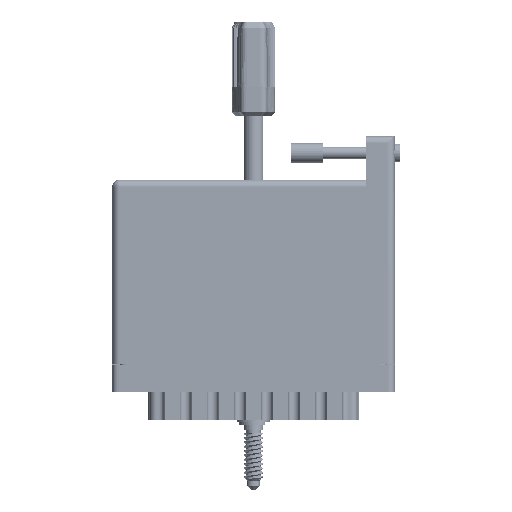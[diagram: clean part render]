
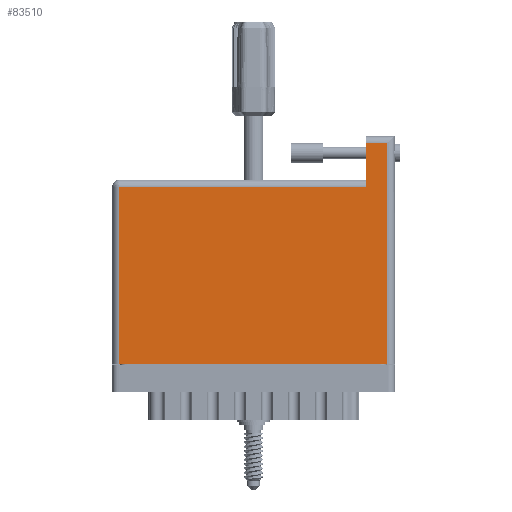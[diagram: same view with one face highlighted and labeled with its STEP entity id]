
A CAD part, front view. The second image highlights one B-rep face of the part: STEP entity #83510.
In plain terms, the highlighted face is planar.
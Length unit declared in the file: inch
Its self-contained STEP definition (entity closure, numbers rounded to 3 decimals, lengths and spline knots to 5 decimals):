
#1133 = VECTOR ( 'NONE', #14040, 39.37008 ) ;
#1445 = CARTESIAN_POINT ( 'NONE',  ( 0.07, 1.705, 0. ) ) ;
#1449 = CARTESIAN_POINT ( 'NONE',  ( 0., 1.775, 0. ) ) ;
#6868 = EDGE_CURVE ( 'NONE', #33301, #13850, #14302, .T. ) ;
#8871 = AXIS2_PLACEMENT_3D ( 'NONE', #1449, #35741, #36329 ) ;
#9872 = LINE ( 'NONE', #56781, #33595 ) ;
#11397 = VECTOR ( 'NONE', #49654, 39.37008 ) ;
#13599 = CARTESIAN_POINT ( 'NONE',  ( 2.438, 2.195, 0. ) ) ;
#13850 = VERTEX_POINT ( 'NONE', #48962 ) ;
#14040 = DIRECTION ( 'NONE',  ( -1., 0., 0. ) ) ;
#14302 = LINE ( 'NONE', #68825, #68151 ) ;
#14479 = EDGE_CURVE ( 'NONE', #65172, #54141, #22150, .T. ) ;
#15605 = ORIENTED_EDGE ( 'NONE', *, *, #6868, .T. ) ;
#17155 = EDGE_CURVE ( 'NONE', #54141, #33301, #9872, .T. ) ;
#19374 = DIRECTION ( 'NONE',  ( 0., 1., 0. ) ) ;
#20775 = ORIENTED_EDGE ( 'NONE', *, *, #49079, .T. ) ;
#22150 = LINE ( 'NONE', #13599, #11397 ) ;
#22291 = ORIENTED_EDGE ( 'NONE', *, *, #17155, .T. ) ;
#32911 = CARTESIAN_POINT ( 'NONE',  ( 2.438, 1.705, 0. ) ) ;
#33004 = ORIENTED_EDGE ( 'NONE', *, *, #87401, .T. ) ;
#33038 = CARTESIAN_POINT ( 'NONE',  ( 2.648, 0., 0. ) ) ;
#33301 = VERTEX_POINT ( 'NONE', #1445 ) ;
#33422 = LINE ( 'NONE', #89007, #1133 ) ;
#33595 = VECTOR ( 'NONE', #64015, 39.37008 ) ;
#35741 = DIRECTION ( 'NONE',  ( 0., 0., -1. ) ) ;
#36329 = DIRECTION ( 'NONE',  ( -1., 0., 0. ) ) ;
#37536 = ORIENTED_EDGE ( 'NONE', *, *, #14479, .T. ) ;
#39173 = CARTESIAN_POINT ( 'NONE',  ( 2.438, 2.125, 0. ) ) ;
#39257 = DIRECTION ( 'NONE',  ( 1., 0., 0. ) ) ;
#43702 = EDGE_CURVE ( 'NONE', #71905, #65172, #33422, .T. ) ;
#46460 = FACE_OUTER_BOUND ( 'NONE', #63848, .T. ) ;
#47483 = LINE ( 'NONE', #61271, #85107 ) ;
#48962 = CARTESIAN_POINT ( 'NONE',  ( 0.07, 0., 0. ) ) ;
#49079 = EDGE_CURVE ( 'NONE', #64079, #71905, #47483, .T. ) ;
#49654 = DIRECTION ( 'NONE',  ( 0., -1., 0. ) ) ;
#53445 = CARTESIAN_POINT ( 'NONE',  ( 0., 0., 0. ) ) ;
#54141 = VERTEX_POINT ( 'NONE', #32911 ) ;
#55409 = CARTESIAN_POINT ( 'NONE',  ( 2.648, 2.125, 0. ) ) ;
#56781 = CARTESIAN_POINT ( 'NONE',  ( 0., 1.705, 0. ) ) ;
#61271 = CARTESIAN_POINT ( 'NONE',  ( 2.648, 2.195, 0. ) ) ;
#61623 = DIRECTION ( 'NONE',  ( 0., -1., 0. ) ) ;
#63848 = EDGE_LOOP ( 'NONE', ( #22291, #15605, #33004, #20775, #87727, #37536 ) ) ;
#64015 = DIRECTION ( 'NONE',  ( -1., 0., 0. ) ) ;
#64079 = VERTEX_POINT ( 'NONE', #33038 ) ;
#65172 = VERTEX_POINT ( 'NONE', #39173 ) ;
#66439 = VECTOR ( 'NONE', #39257, 39.37008 ) ;
#68151 = VECTOR ( 'NONE', #61623, 39.37008 ) ;
#68825 = CARTESIAN_POINT ( 'NONE',  ( 0.07, 0., 0. ) ) ;
#70097 = PLANE ( 'NONE',  #8871 ) ;
#71905 = VERTEX_POINT ( 'NONE', #55409 ) ;
#76100 = LINE ( 'NONE', #53445, #66439 ) ;
#83510 = ADVANCED_FACE ( 'NONE', ( #46460 ), #70097, .F. ) ;
#85107 = VECTOR ( 'NONE', #19374, 39.37008 ) ;
#87401 = EDGE_CURVE ( 'NONE', #13850, #64079, #76100, .T. ) ;
#87727 = ORIENTED_EDGE ( 'NONE', *, *, #43702, .T. ) ;
#89007 = CARTESIAN_POINT ( 'NONE',  ( 0., 2.125, 0. ) ) ;
